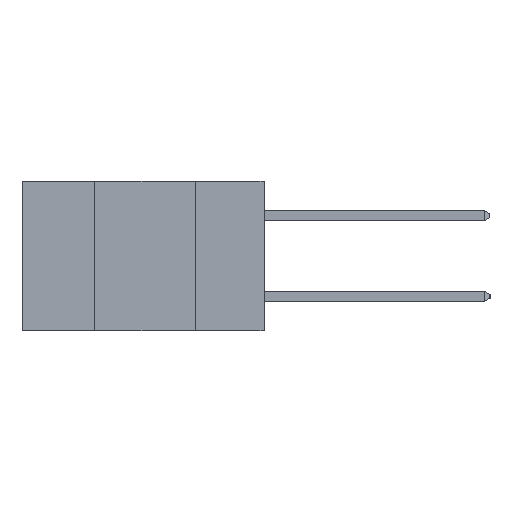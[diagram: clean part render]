
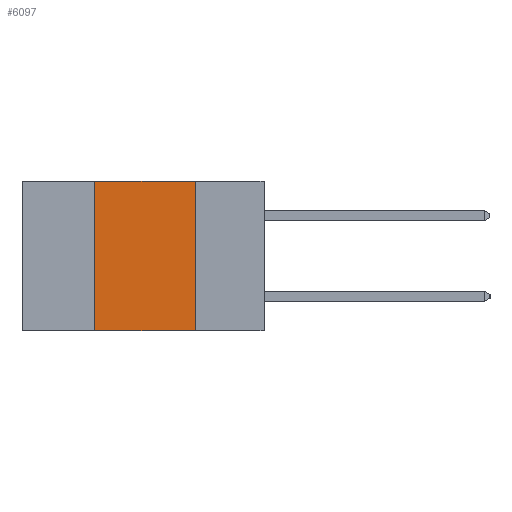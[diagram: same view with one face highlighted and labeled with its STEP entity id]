
A CAD part, left-side view. The second image highlights one B-rep face of the part: STEP entity #6097.
In plain terms, the highlighted planar face has unit normal (-1, 0, 0).
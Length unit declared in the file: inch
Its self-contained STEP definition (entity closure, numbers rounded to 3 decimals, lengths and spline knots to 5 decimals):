
#833 = LINE ( 'NONE', #5620, #8469 ) ;
#1499 = CARTESIAN_POINT ( 'NONE',  ( 0., 0.17, -0.37 ) ) ;
#1550 = LINE ( 'NONE', #8619, #9361 ) ;
#1721 = VERTEX_POINT ( 'NONE', #8515 ) ;
#1940 = VECTOR ( 'NONE', #4935, 39.37008 ) ;
#2137 = EDGE_CURVE ( 'NONE', #3649, #2958, #3910, .T. ) ;
#2344 = ORIENTED_EDGE ( 'NONE', *, *, #2137, .F. ) ;
#2958 = VERTEX_POINT ( 'NONE', #7620 ) ;
#3239 = EDGE_CURVE ( 'NONE', #3649, #8023, #833, .T. ) ;
#3395 = DIRECTION ( 'NONE',  ( 0., -1., 0. ) ) ;
#3429 = CARTESIAN_POINT ( 'NONE',  ( 0., 0.17, -0.37 ) ) ;
#3649 = VERTEX_POINT ( 'NONE', #7569 ) ;
#3902 = DIRECTION ( 'NONE',  ( 1., 0., 0. ) ) ;
#3910 = LINE ( 'NONE', #5317, #7900 ) ;
#4927 = EDGE_LOOP ( 'NONE', ( #5891, #9689, #2344, #7098 ) ) ;
#4935 = DIRECTION ( 'NONE',  ( 0., 0., -1. ) ) ;
#5317 = CARTESIAN_POINT ( 'NONE',  ( 0., 0.42, -0.37 ) ) ;
#5620 = CARTESIAN_POINT ( 'NONE',  ( 0., 0.6, -0.37 ) ) ;
#5839 = DIRECTION ( 'NONE',  ( 0., 0., 1. ) ) ;
#5891 = ORIENTED_EDGE ( 'NONE', *, *, #9096, .F. ) ;
#5970 = LINE ( 'NONE', #3429, #1940 ) ;
#6097 = ADVANCED_FACE ( 'NONE', ( #7953 ), #8399, .F. ) ;
#7098 = ORIENTED_EDGE ( 'NONE', *, *, #3239, .T. ) ;
#7131 = DIRECTION ( 'NONE',  ( 0., -1., 0. ) ) ;
#7569 = CARTESIAN_POINT ( 'NONE',  ( 0., 0.42, -0.37 ) ) ;
#7620 = CARTESIAN_POINT ( 'NONE',  ( 0., 0.42, 0. ) ) ;
#7784 = AXIS2_PLACEMENT_3D ( 'NONE', #9841, #3902, #9149 ) ;
#7900 = VECTOR ( 'NONE', #5839, 39.37008 ) ;
#7953 = FACE_OUTER_BOUND ( 'NONE', #4927, .T. ) ;
#8023 = VERTEX_POINT ( 'NONE', #1499 ) ;
#8399 = PLANE ( 'NONE',  #7784 ) ;
#8469 = VECTOR ( 'NONE', #3395, 39.37008 ) ;
#8515 = CARTESIAN_POINT ( 'NONE',  ( 0., 0.17, 0. ) ) ;
#8619 = CARTESIAN_POINT ( 'NONE',  ( 0., 0.6, 0. ) ) ;
#8899 = EDGE_CURVE ( 'NONE', #2958, #1721, #1550, .T. ) ;
#9096 = EDGE_CURVE ( 'NONE', #1721, #8023, #5970, .T. ) ;
#9149 = DIRECTION ( 'NONE',  ( 0., 0., -1. ) ) ;
#9361 = VECTOR ( 'NONE', #7131, 39.37008 ) ;
#9689 = ORIENTED_EDGE ( 'NONE', *, *, #8899, .F. ) ;
#9841 = CARTESIAN_POINT ( 'NONE',  ( 0., 0.6, 0. ) ) ;
